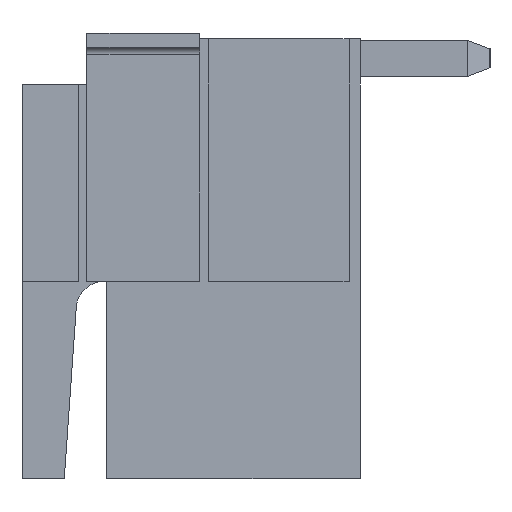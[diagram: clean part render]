
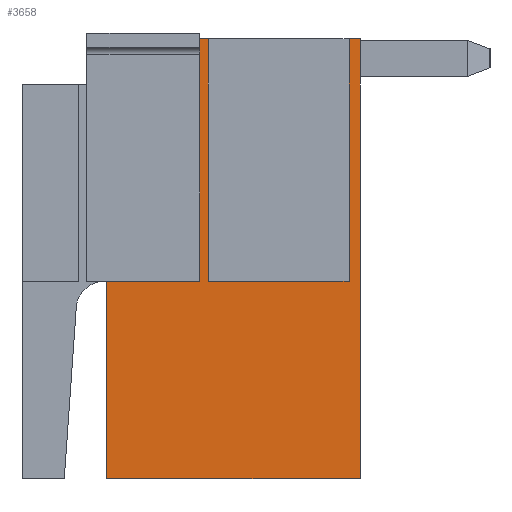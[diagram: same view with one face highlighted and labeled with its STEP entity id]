
A CAD part, left-side view. The second image highlights one B-rep face of the part: STEP entity #3658.
In plain terms, the highlighted planar face has unit normal (-1, 0, 0).
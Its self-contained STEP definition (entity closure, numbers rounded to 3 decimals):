
#86 = ORIENTED_EDGE ( 'NONE', *, *, #5995, .T. ) ;
#142 = DIRECTION ( 'NONE',  ( 0., 0., -1. ) ) ;
#158 = VERTEX_POINT ( 'NONE', #4367 ) ;
#183 = VECTOR ( 'NONE', #3748, 1000. ) ;
#239 = EDGE_CURVE ( 'NONE', #1847, #1973, #6003, .T. ) ;
#380 = CARTESIAN_POINT ( 'NONE',  ( -7.5, 0., 0. ) ) ;
#530 = VERTEX_POINT ( 'NONE', #2743 ) ;
#607 = CARTESIAN_POINT ( 'NONE',  ( -7.5, -3.1, -3.9 ) ) ;
#624 = DIRECTION ( 'NONE',  ( 0., 1., 0. ) ) ;
#660 = CARTESIAN_POINT ( 'NONE',  ( -7.5, -2.9, -0.4 ) ) ;
#736 = DIRECTION ( 'NONE',  ( 0., -1., 0. ) ) ;
#820 = CARTESIAN_POINT ( 'NONE',  ( -7.5, 1.4, -0.4 ) ) ;
#840 = ORIENTED_EDGE ( 'NONE', *, *, #239, .T. ) ;
#947 = VERTEX_POINT ( 'NONE', #3099 ) ;
#948 = AXIS2_PLACEMENT_3D ( 'NONE', #380, #3082, #3600 ) ;
#1054 = LINE ( 'NONE', #4339, #2964 ) ;
#1088 = EDGE_CURVE ( 'NONE', #1454, #530, #4406, .T. ) ;
#1116 = VERTEX_POINT ( 'NONE', #1715 ) ;
#1209 = VECTOR ( 'NONE', #6494, 1000. ) ;
#1216 = CARTESIAN_POINT ( 'NONE',  ( -7.5, -3.1, -5.067 ) ) ;
#1282 = DIRECTION ( 'NONE',  ( 0., 0., 1. ) ) ;
#1336 = CARTESIAN_POINT ( 'NONE',  ( -7.5, -2.9, -0.4 ) ) ;
#1343 = LINE ( 'NONE', #1407, #3218 ) ;
#1407 = CARTESIAN_POINT ( 'NONE',  ( -7.5, -2.9, -3.195 ) ) ;
#1454 = VERTEX_POINT ( 'NONE', #820 ) ;
#1491 = LINE ( 'NONE', #5751, #3199 ) ;
#1538 = CARTESIAN_POINT ( 'NONE',  ( -7.5, 1.15, 3.9 ) ) ;
#1660 = ORIENTED_EDGE ( 'NONE', *, *, #2139, .F. ) ;
#1672 = CARTESIAN_POINT ( 'NONE',  ( -7.5, -0.4, -3.195 ) ) ;
#1715 = CARTESIAN_POINT ( 'NONE',  ( -7.5, -2.9, 3.9 ) ) ;
#1766 = CARTESIAN_POINT ( 'NONE',  ( -7.5, 1.15, 3.9 ) ) ;
#1810 = CARTESIAN_POINT ( 'NONE',  ( -7.5, -2.9, -3.9 ) ) ;
#1840 = EDGE_LOOP ( 'NONE', ( #2447, #2569, #6104, #3372, #86, #6567, #3220, #840, #2165, #6257, #1660, #4496 ) ) ;
#1847 = VERTEX_POINT ( 'NONE', #1336 ) ;
#1973 = VERTEX_POINT ( 'NONE', #6888 ) ;
#2139 = EDGE_CURVE ( 'NONE', #947, #2399, #1054, .T. ) ;
#2165 = ORIENTED_EDGE ( 'NONE', *, *, #5449, .T. ) ;
#2241 = LINE ( 'NONE', #4369, #3741 ) ;
#2261 = CARTESIAN_POINT ( 'NONE',  ( -7.5, 1.15, 3.9 ) ) ;
#2396 = VECTOR ( 'NONE', #6638, 1000. ) ;
#2399 = VERTEX_POINT ( 'NONE', #1538 ) ;
#2447 = ORIENTED_EDGE ( 'NONE', *, *, #2754, .F. ) ;
#2526 = CARTESIAN_POINT ( 'NONE',  ( -7.5, -0.4, 3.9 ) ) ;
#2569 = ORIENTED_EDGE ( 'NONE', *, *, #1088, .F. ) ;
#2634 = LINE ( 'NONE', #3699, #3813 ) ;
#2743 = CARTESIAN_POINT ( 'NONE',  ( -7.5, -0.25, -0.4 ) ) ;
#2754 = EDGE_CURVE ( 'NONE', #530, #6562, #1491, .T. ) ;
#2964 = VECTOR ( 'NONE', #3193, 1000. ) ;
#3082 = DIRECTION ( 'NONE',  ( 1., 0., 0. ) ) ;
#3099 = CARTESIAN_POINT ( 'NONE',  ( -7.5, 1.166, 3.875 ) ) ;
#3118 = VECTOR ( 'NONE', #624, 1000. ) ;
#3193 = DIRECTION ( 'NONE',  ( 0., -0.53, 0.848 ) ) ;
#3199 = VECTOR ( 'NONE', #3627, 1000. ) ;
#3218 = VECTOR ( 'NONE', #5600, 1000. ) ;
#3220 = ORIENTED_EDGE ( 'NONE', *, *, #6655, .F. ) ;
#3372 = ORIENTED_EDGE ( 'NONE', *, *, #3550, .F. ) ;
#3422 = EDGE_CURVE ( 'NONE', #1454, #158, #2241, .T. ) ;
#3458 = LINE ( 'NONE', #1216, #4650 ) ;
#3550 = EDGE_CURVE ( 'NONE', #6279, #158, #6604, .T. ) ;
#3600 = DIRECTION ( 'NONE',  ( 0., 0., -1. ) ) ;
#3627 = DIRECTION ( 'NONE',  ( 0., 0., 1. ) ) ;
#3658 = ADVANCED_FACE ( 'NONE', ( #4645 ), #5757, .F. ) ;
#3699 = CARTESIAN_POINT ( 'NONE',  ( -7.5, 1.75, 3.875 ) ) ;
#3741 = VECTOR ( 'NONE', #142, 1000. ) ;
#3748 = DIRECTION ( 'NONE',  ( 0., 0., 1. ) ) ;
#3813 = VECTOR ( 'NONE', #5355, 1000. ) ;
#4057 = VERTEX_POINT ( 'NONE', #4082 ) ;
#4082 = CARTESIAN_POINT ( 'NONE',  ( -7.5, -3.1, 3.9 ) ) ;
#4338 = EDGE_CURVE ( 'NONE', #2399, #4960, #5050, .T. ) ;
#4339 = CARTESIAN_POINT ( 'NONE',  ( -7.5, 1.65, 3.1 ) ) ;
#4367 = CARTESIAN_POINT ( 'NONE',  ( -7.5, 1.4, -3.9 ) ) ;
#4368 = LINE ( 'NONE', #1672, #183 ) ;
#4369 = CARTESIAN_POINT ( 'NONE',  ( -7.5, 1.4, -3.9 ) ) ;
#4377 = EDGE_CURVE ( 'NONE', #1116, #4057, #5496, .T. ) ;
#4406 = LINE ( 'NONE', #5379, #5336 ) ;
#4496 = ORIENTED_EDGE ( 'NONE', *, *, #4658, .T. ) ;
#4645 = FACE_OUTER_BOUND ( 'NONE', #1840, .T. ) ;
#4650 = VECTOR ( 'NONE', #1282, 1000. ) ;
#4658 = EDGE_CURVE ( 'NONE', #947, #6562, #2634, .T. ) ;
#4960 = VERTEX_POINT ( 'NONE', #2526 ) ;
#5050 = LINE ( 'NONE', #2261, #6566 ) ;
#5336 = VECTOR ( 'NONE', #736, 1000. ) ;
#5355 = DIRECTION ( 'NONE',  ( 0., -1., 0. ) ) ;
#5379 = CARTESIAN_POINT ( 'NONE',  ( -7.5, 1.75, -0.4 ) ) ;
#5449 = EDGE_CURVE ( 'NONE', #1973, #4960, #4368, .T. ) ;
#5466 = DIRECTION ( 'NONE',  ( 0., -1., 0. ) ) ;
#5496 = LINE ( 'NONE', #1766, #1209 ) ;
#5600 = DIRECTION ( 'NONE',  ( 0., 0., 1. ) ) ;
#5751 = CARTESIAN_POINT ( 'NONE',  ( -7.5, -0.25, -0.4 ) ) ;
#5757 = PLANE ( 'NONE',  #948 ) ;
#5995 = EDGE_CURVE ( 'NONE', #6279, #4057, #3458, .T. ) ;
#6003 = LINE ( 'NONE', #660, #3118 ) ;
#6104 = ORIENTED_EDGE ( 'NONE', *, *, #3422, .T. ) ;
#6195 = CARTESIAN_POINT ( 'NONE',  ( -7.5, -0.25, 3.875 ) ) ;
#6257 = ORIENTED_EDGE ( 'NONE', *, *, #4338, .F. ) ;
#6279 = VERTEX_POINT ( 'NONE', #607 ) ;
#6494 = DIRECTION ( 'NONE',  ( 0., -1., 0. ) ) ;
#6562 = VERTEX_POINT ( 'NONE', #6195 ) ;
#6566 = VECTOR ( 'NONE', #5466, 1000. ) ;
#6567 = ORIENTED_EDGE ( 'NONE', *, *, #4377, .F. ) ;
#6604 = LINE ( 'NONE', #1810, #2396 ) ;
#6638 = DIRECTION ( 'NONE',  ( 0., 1., 0. ) ) ;
#6655 = EDGE_CURVE ( 'NONE', #1847, #1116, #1343, .T. ) ;
#6888 = CARTESIAN_POINT ( 'NONE',  ( -7.5, -0.4, -0.4 ) ) ;
